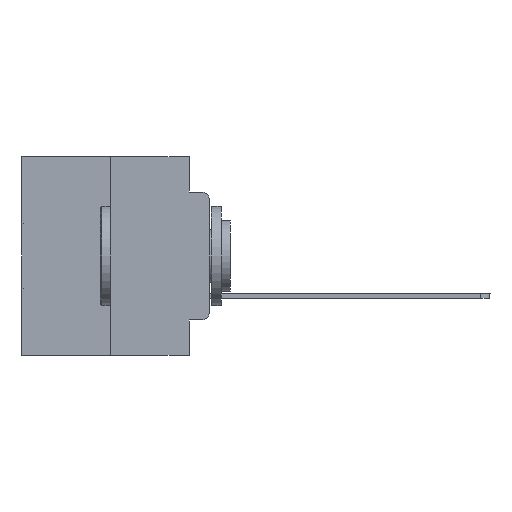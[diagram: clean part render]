
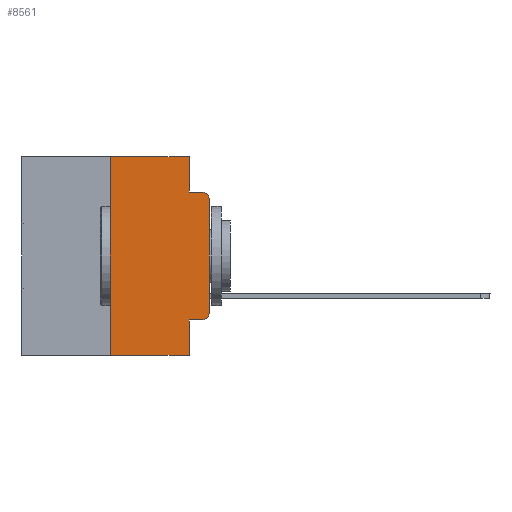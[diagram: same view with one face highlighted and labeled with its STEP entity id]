
A CAD part, left-side view. The second image highlights one B-rep face of the part: STEP entity #8561.
In plain terms, the highlighted planar face has unit normal (-1, 0, 0).
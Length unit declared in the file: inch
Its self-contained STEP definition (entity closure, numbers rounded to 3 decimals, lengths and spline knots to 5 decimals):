
#227 = VERTEX_POINT ( 'NONE', #17807 ) ;
#843 = EDGE_CURVE ( 'NONE', #14856, #28311, #8540, .T. ) ;
#886 = EDGE_CURVE ( 'NONE', #227, #24407, #3616, .T. ) ;
#1220 = VECTOR ( 'NONE', #8940, 39.37008 ) ;
#1570 = PLANE ( 'NONE',  #13786 ) ;
#1874 = LINE ( 'NONE', #17981, #19020 ) ;
#1924 = DIRECTION ( 'NONE',  ( 0., 0., -1. ) ) ;
#1931 = VECTOR ( 'NONE', #7055, 39.37008 ) ;
#2609 = CARTESIAN_POINT ( 'NONE',  ( 0., 0.02, -0.0885 ) ) ;
#3616 = LINE ( 'NONE', #27259, #19733 ) ;
#4743 = DIRECTION ( 'NONE',  ( 0., 0., 1. ) ) ;
#4824 = DIRECTION ( 'NONE',  ( 0., -1., 0. ) ) ;
#4962 = DIRECTION ( 'NONE',  ( 0., -1., 0. ) ) ;
#5666 = EDGE_CURVE ( 'NONE', #15740, #13283, #21124, .T. ) ;
#5717 = EDGE_LOOP ( 'NONE', ( #26293, #13978, #7072, #14727, #20814, #28062, #18701, #23794, #22939, #13789 ) ) ;
#5745 = AXIS2_PLACEMENT_3D ( 'NONE', #10967, #21871, #24773 ) ;
#6234 = CARTESIAN_POINT ( 'NONE',  ( 0., 0.473, 0. ) ) ;
#6306 = LINE ( 'NONE', #11878, #18206 ) ;
#6506 = AXIS2_PLACEMENT_3D ( 'NONE', #6591, #28743, #1924 ) ;
#6591 = CARTESIAN_POINT ( 'NONE',  ( 0., 0.02, -0.3915 ) ) ;
#6754 = VECTOR ( 'NONE', #18228, 39.37008 ) ;
#7018 = LINE ( 'NONE', #9587, #7344 ) ;
#7055 = DIRECTION ( 'NONE',  ( 0., 0., 1. ) ) ;
#7072 = ORIENTED_EDGE ( 'NONE', *, *, #24514, .F. ) ;
#7244 = DIRECTION ( 'NONE',  ( 0., 0., -1. ) ) ;
#7344 = VECTOR ( 'NONE', #4962, 39.37008 ) ;
#7901 = VERTEX_POINT ( 'NONE', #2609 ) ;
#8011 = CIRCLE ( 'NONE', #5745, 0.02 ) ;
#8540 = CIRCLE ( 'NONE', #6506, 0.02 ) ;
#8561 = ADVANCED_FACE ( 'NONE', ( #22000 ), #1570, .F. ) ;
#8940 = DIRECTION ( 'NONE',  ( 0., -1., 0. ) ) ;
#9087 = CARTESIAN_POINT ( 'NONE',  ( 0., 0.051, -0.0885 ) ) ;
#9587 = CARTESIAN_POINT ( 'NONE',  ( 0., 0.051, -0.0885 ) ) ;
#10237 = EDGE_CURVE ( 'NONE', #13122, #7901, #8011, .T. ) ;
#10846 = EDGE_CURVE ( 'NONE', #227, #13283, #15038, .T. ) ;
#10967 = CARTESIAN_POINT ( 'NONE',  ( 0., 0.02, -0.1085 ) ) ;
#11878 = CARTESIAN_POINT ( 'NONE',  ( 0., 0.051, 0. ) ) ;
#12653 = DIRECTION ( 'NONE',  ( 1., 0., 0. ) ) ;
#13122 = VERTEX_POINT ( 'NONE', #24109 ) ;
#13283 = VERTEX_POINT ( 'NONE', #19920 ) ;
#13786 = AXIS2_PLACEMENT_3D ( 'NONE', #6234, #12653, #28303 ) ;
#13789 = ORIENTED_EDGE ( 'NONE', *, *, #843, .T. ) ;
#13978 = ORIENTED_EDGE ( 'NONE', *, *, #10237, .T. ) ;
#14034 = CARTESIAN_POINT ( 'NONE',  ( 0., 0., 0. ) ) ;
#14063 = CARTESIAN_POINT ( 'NONE',  ( 0., 0., -0.3915 ) ) ;
#14576 = VERTEX_POINT ( 'NONE', #9087 ) ;
#14727 = ORIENTED_EDGE ( 'NONE', *, *, #28886, .F. ) ;
#14856 = VERTEX_POINT ( 'NONE', #19134 ) ;
#15038 = LINE ( 'NONE', #24894, #24121 ) ;
#15625 = CARTESIAN_POINT ( 'NONE',  ( 0., 0.051, -0.4115 ) ) ;
#15740 = VERTEX_POINT ( 'NONE', #15625 ) ;
#17807 = CARTESIAN_POINT ( 'NONE',  ( 0., 0.25, -0.5 ) ) ;
#17981 = CARTESIAN_POINT ( 'NONE',  ( 0., 0.051, -0.4115 ) ) ;
#18076 = DIRECTION ( 'NONE',  ( 0., -1., 0. ) ) ;
#18206 = VECTOR ( 'NONE', #7244, 39.37008 ) ;
#18228 = DIRECTION ( 'NONE',  ( 0., 0., -1. ) ) ;
#18701 = ORIENTED_EDGE ( 'NONE', *, *, #10846, .T. ) ;
#19020 = VECTOR ( 'NONE', #18076, 39.37008 ) ;
#19077 = LINE ( 'NONE', #14034, #1931 ) ;
#19134 = CARTESIAN_POINT ( 'NONE',  ( 0., 0.02, -0.4115 ) ) ;
#19733 = VECTOR ( 'NONE', #4743, 39.37008 ) ;
#19920 = CARTESIAN_POINT ( 'NONE',  ( 0., 0.051, -0.5 ) ) ;
#20167 = CARTESIAN_POINT ( 'NONE',  ( 0., 0.25, 0. ) ) ;
#20428 = CARTESIAN_POINT ( 'NONE',  ( 0., 0.051, 0. ) ) ;
#20814 = ORIENTED_EDGE ( 'NONE', *, *, #21502, .F. ) ;
#20849 = LINE ( 'NONE', #28797, #1220 ) ;
#21124 = LINE ( 'NONE', #22941, #6754 ) ;
#21502 = EDGE_CURVE ( 'NONE', #24407, #23207, #20849, .T. ) ;
#21871 = DIRECTION ( 'NONE',  ( -1., 0., 0. ) ) ;
#22000 = FACE_OUTER_BOUND ( 'NONE', #5717, .T. ) ;
#22199 = EDGE_CURVE ( 'NONE', #28311, #13122, #19077, .T. ) ;
#22939 = ORIENTED_EDGE ( 'NONE', *, *, #23247, .T. ) ;
#22941 = CARTESIAN_POINT ( 'NONE',  ( 0., 0.051, 0. ) ) ;
#23207 = VERTEX_POINT ( 'NONE', #20428 ) ;
#23247 = EDGE_CURVE ( 'NONE', #15740, #14856, #1874, .T. ) ;
#23794 = ORIENTED_EDGE ( 'NONE', *, *, #5666, .F. ) ;
#24109 = CARTESIAN_POINT ( 'NONE',  ( 0., 0., -0.1085 ) ) ;
#24121 = VECTOR ( 'NONE', #4824, 39.37008 ) ;
#24407 = VERTEX_POINT ( 'NONE', #20167 ) ;
#24514 = EDGE_CURVE ( 'NONE', #14576, #7901, #7018, .T. ) ;
#24773 = DIRECTION ( 'NONE',  ( 0., 0., -1. ) ) ;
#24894 = CARTESIAN_POINT ( 'NONE',  ( 0., 0.473, -0.5 ) ) ;
#26293 = ORIENTED_EDGE ( 'NONE', *, *, #22199, .T. ) ;
#27259 = CARTESIAN_POINT ( 'NONE',  ( 0., 0.25, 0. ) ) ;
#28062 = ORIENTED_EDGE ( 'NONE', *, *, #886, .F. ) ;
#28303 = DIRECTION ( 'NONE',  ( 0., 0., -1. ) ) ;
#28311 = VERTEX_POINT ( 'NONE', #14063 ) ;
#28743 = DIRECTION ( 'NONE',  ( -1., 0., 0. ) ) ;
#28797 = CARTESIAN_POINT ( 'NONE',  ( 0., 0.473, 0. ) ) ;
#28886 = EDGE_CURVE ( 'NONE', #23207, #14576, #6306, .T. ) ;
